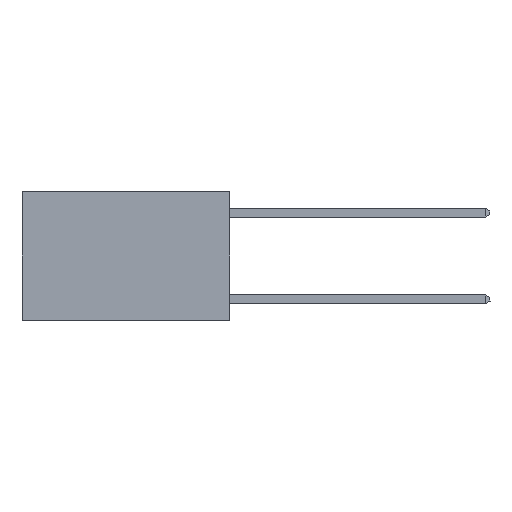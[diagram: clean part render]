
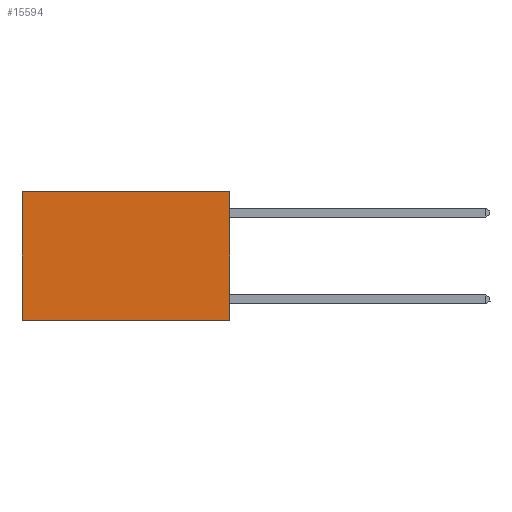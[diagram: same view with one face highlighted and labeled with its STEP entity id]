
A CAD part, left-side view. The second image highlights one B-rep face of the part: STEP entity #15594.
In plain terms, the highlighted planar face has unit normal (-1, 0, 0).
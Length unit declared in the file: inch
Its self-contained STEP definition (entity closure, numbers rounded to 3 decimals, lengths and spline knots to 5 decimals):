
#464 = CARTESIAN_POINT ( 'NONE',  ( 0.2625, 0., 0. ) ) ;
#526 = PLANE ( 'NONE',  #18647 ) ;
#1580 = VECTOR ( 'NONE', #17599, 39.37008 ) ;
#1744 = EDGE_CURVE ( 'NONE', #13278, #11339, #19100, .T. ) ;
#2183 = CARTESIAN_POINT ( 'NONE',  ( 0.2625, 0., 0. ) ) ;
#2529 = CARTESIAN_POINT ( 'NONE',  ( 0.2625, 0.6, 0. ) ) ;
#3944 = FACE_OUTER_BOUND ( 'NONE', #5685, .T. ) ;
#4098 = ORIENTED_EDGE ( 'NONE', *, *, #1744, .T. ) ;
#4189 = DIRECTION ( 'NONE',  ( 0., 0., -1. ) ) ;
#4632 = CARTESIAN_POINT ( 'NONE',  ( 0.2625, 0.6, 0. ) ) ;
#5467 = VERTEX_POINT ( 'NONE', #2183 ) ;
#5481 = VECTOR ( 'NONE', #11699, 39.37008 ) ;
#5685 = EDGE_LOOP ( 'NONE', ( #4098, #18137, #5962, #13103 ) ) ;
#5962 = ORIENTED_EDGE ( 'NONE', *, *, #7110, .F. ) ;
#6331 = CARTESIAN_POINT ( 'NONE',  ( 0.2625, 0.6, -0.37 ) ) ;
#6709 = DIRECTION ( 'NONE',  ( 1., 0., 0. ) ) ;
#7110 = EDGE_CURVE ( 'NONE', #5467, #8928, #7447, .T. ) ;
#7121 = CARTESIAN_POINT ( 'NONE',  ( 0.2625, 0., -0.37 ) ) ;
#7447 = LINE ( 'NONE', #464, #18456 ) ;
#7468 = LINE ( 'NONE', #7121, #1580 ) ;
#8020 = DIRECTION ( 'NONE',  ( 0., 0., -1. ) ) ;
#8928 = VERTEX_POINT ( 'NONE', #13277 ) ;
#11339 = VERTEX_POINT ( 'NONE', #6331 ) ;
#11368 = VECTOR ( 'NONE', #4189, 39.37008 ) ;
#11699 = DIRECTION ( 'NONE',  ( 0., 1., 0. ) ) ;
#11743 = EDGE_CURVE ( 'NONE', #5467, #13278, #13700, .T. ) ;
#13103 = ORIENTED_EDGE ( 'NONE', *, *, #11743, .T. ) ;
#13277 = CARTESIAN_POINT ( 'NONE',  ( 0.2625, 0., -0.37 ) ) ;
#13278 = VERTEX_POINT ( 'NONE', #4632 ) ;
#13700 = LINE ( 'NONE', #17709, #5481 ) ;
#15169 = EDGE_CURVE ( 'NONE', #8928, #11339, #7468, .T. ) ;
#15594 = ADVANCED_FACE ( 'NONE', ( #3944 ), #526, .F. ) ;
#15680 = CARTESIAN_POINT ( 'NONE',  ( 0.2625, 0., 0. ) ) ;
#17167 = DIRECTION ( 'NONE',  ( 0., 0., -1. ) ) ;
#17599 = DIRECTION ( 'NONE',  ( 0., 1., 0. ) ) ;
#17709 = CARTESIAN_POINT ( 'NONE',  ( 0.2625, 0., 0. ) ) ;
#18137 = ORIENTED_EDGE ( 'NONE', *, *, #15169, .F. ) ;
#18456 = VECTOR ( 'NONE', #8020, 39.37008 ) ;
#18647 = AXIS2_PLACEMENT_3D ( 'NONE', #15680, #6709, #17167 ) ;
#19100 = LINE ( 'NONE', #2529, #11368 ) ;
